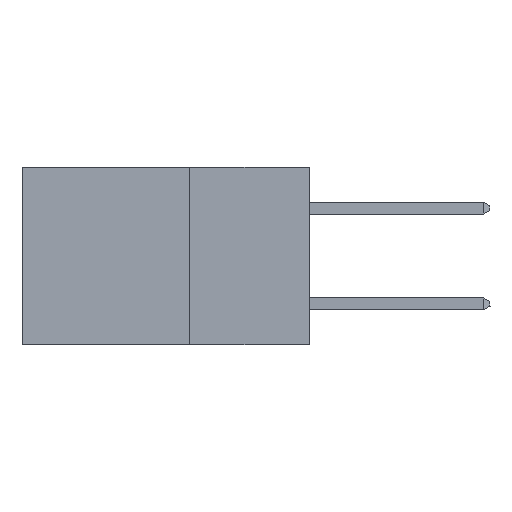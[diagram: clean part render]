
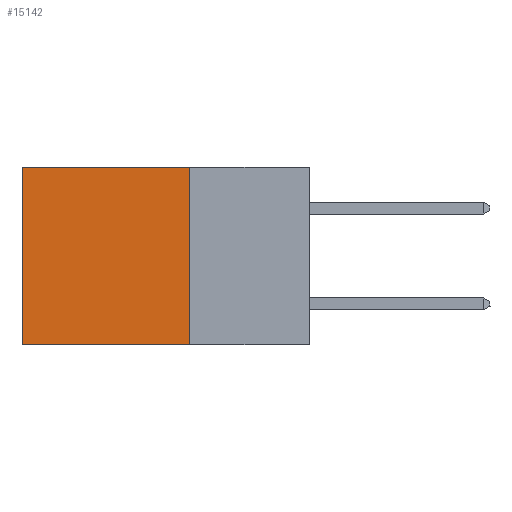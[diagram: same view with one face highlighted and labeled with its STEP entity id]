
A CAD part, left-side view. The second image highlights one B-rep face of the part: STEP entity #15142.
In plain terms, the highlighted planar face has unit normal (-1, 0, 0).
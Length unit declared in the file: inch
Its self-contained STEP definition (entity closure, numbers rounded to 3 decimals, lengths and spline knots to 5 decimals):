
#814 = EDGE_CURVE ( 'NONE', #14083, #1069, #1309, .T. ) ;
#974 = EDGE_CURVE ( 'NONE', #19167, #14083, #10672, .T. ) ;
#1069 = VERTEX_POINT ( 'NONE', #6000 ) ;
#1309 = LINE ( 'NONE', #12711, #5090 ) ;
#2332 = ORIENTED_EDGE ( 'NONE', *, *, #5342, .F. ) ;
#2758 = VECTOR ( 'NONE', #16478, 39.37008 ) ;
#2796 = PLANE ( 'NONE',  #18874 ) ;
#4420 = DIRECTION ( 'NONE',  ( 0., 0., -1. ) ) ;
#5090 = VECTOR ( 'NONE', #12853, 39.37008 ) ;
#5203 = EDGE_CURVE ( 'NONE', #19167, #17537, #15110, .T. ) ;
#5342 = EDGE_CURVE ( 'NONE', #17537, #1069, #8878, .T. ) ;
#6000 = CARTESIAN_POINT ( 'NONE',  ( 0.2875, 0.6, -0.37 ) ) ;
#6821 = VECTOR ( 'NONE', #16482, 39.37008 ) ;
#8878 = LINE ( 'NONE', #12003, #16902 ) ;
#10672 = LINE ( 'NONE', #11411, #6821 ) ;
#10783 = CARTESIAN_POINT ( 'NONE',  ( 0.2875, 0.25, 0. ) ) ;
#11411 = CARTESIAN_POINT ( 'NONE',  ( 0.2875, 0.25, 0. ) ) ;
#12003 = CARTESIAN_POINT ( 'NONE',  ( 0.2875, 0.25, -0.37 ) ) ;
#12711 = CARTESIAN_POINT ( 'NONE',  ( 0.2875, 0.6, 0. ) ) ;
#12853 = DIRECTION ( 'NONE',  ( 0., 0., -1. ) ) ;
#13101 = CARTESIAN_POINT ( 'NONE',  ( 0.2875, 0.25, -0.37 ) ) ;
#13105 = FACE_OUTER_BOUND ( 'NONE', #18651, .T. ) ;
#13137 = ORIENTED_EDGE ( 'NONE', *, *, #5203, .F. ) ;
#13570 = DIRECTION ( 'NONE',  ( 0., 1., 0. ) ) ;
#14038 = DIRECTION ( 'NONE',  ( 1., 0., 0. ) ) ;
#14083 = VERTEX_POINT ( 'NONE', #16370 ) ;
#15110 = LINE ( 'NONE', #19614, #2758 ) ;
#15142 = ADVANCED_FACE ( 'NONE', ( #13105 ), #2796, .F. ) ;
#16289 = ORIENTED_EDGE ( 'NONE', *, *, #814, .T. ) ;
#16370 = CARTESIAN_POINT ( 'NONE',  ( 0.2875, 0.6, 0. ) ) ;
#16478 = DIRECTION ( 'NONE',  ( 0., 0., -1. ) ) ;
#16482 = DIRECTION ( 'NONE',  ( 0., 1., 0. ) ) ;
#16902 = VECTOR ( 'NONE', #13570, 39.37008 ) ;
#17537 = VERTEX_POINT ( 'NONE', #13101 ) ;
#18150 = ORIENTED_EDGE ( 'NONE', *, *, #974, .T. ) ;
#18651 = EDGE_LOOP ( 'NONE', ( #16289, #2332, #13137, #18150 ) ) ;
#18874 = AXIS2_PLACEMENT_3D ( 'NONE', #20335, #14038, #4420 ) ;
#19167 = VERTEX_POINT ( 'NONE', #10783 ) ;
#19614 = CARTESIAN_POINT ( 'NONE',  ( 0.2875, 0.25, 0. ) ) ;
#20335 = CARTESIAN_POINT ( 'NONE',  ( 0.2875, 0.25, 0. ) ) ;
